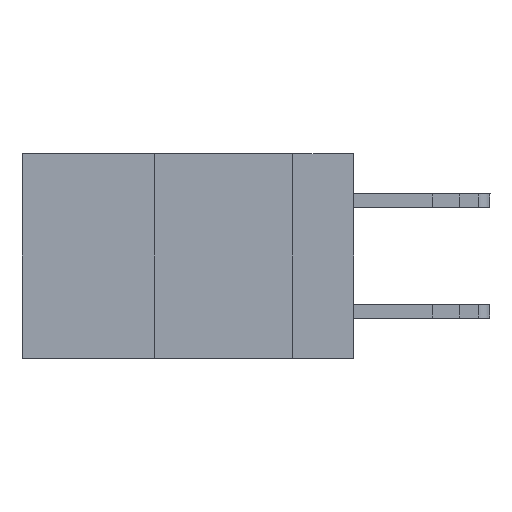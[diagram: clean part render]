
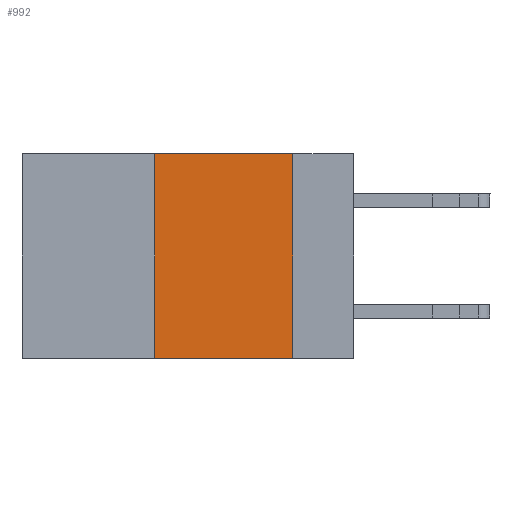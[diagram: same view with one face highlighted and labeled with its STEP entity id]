
A CAD part, left-side view. The second image highlights one B-rep face of the part: STEP entity #992.
In plain terms, the highlighted planar face has unit normal (-1, 0, 0).
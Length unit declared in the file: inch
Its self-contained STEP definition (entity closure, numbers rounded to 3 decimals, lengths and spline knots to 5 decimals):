
#744 = CARTESIAN_POINT ( 'NONE',  ( 0., 0.6, 0. ) ) ;
#855 = VERTEX_POINT ( 'NONE', #23430 ) ;
#992 = ADVANCED_FACE ( 'NONE', ( #20292 ), #3676, .F. ) ;
#1057 = LINE ( 'NONE', #10386, #12485 ) ;
#1118 = EDGE_CURVE ( 'NONE', #20044, #12864, #6195, .T. ) ;
#3676 = PLANE ( 'NONE',  #14341 ) ;
#4461 = LINE ( 'NONE', #11482, #5507 ) ;
#4913 = EDGE_CURVE ( 'NONE', #12864, #23146, #6655, .T. ) ;
#5507 = VECTOR ( 'NONE', #13796, 39.37008 ) ;
#6195 = LINE ( 'NONE', #744, #15088 ) ;
#6655 = LINE ( 'NONE', #12475, #9966 ) ;
#8420 = ORIENTED_EDGE ( 'NONE', *, *, #4913, .F. ) ;
#9239 = DIRECTION ( 'NONE',  ( 0., 0., -1. ) ) ;
#9966 = VECTOR ( 'NONE', #14059, 39.37008 ) ;
#10386 = CARTESIAN_POINT ( 'NONE',  ( 0., 0.36, 0. ) ) ;
#11059 = DIRECTION ( 'NONE',  ( 1., 0., 0. ) ) ;
#11482 = CARTESIAN_POINT ( 'NONE',  ( 0., 0.6, -0.37 ) ) ;
#11906 = EDGE_CURVE ( 'NONE', #855, #20044, #1057, .T. ) ;
#12475 = CARTESIAN_POINT ( 'NONE',  ( 0., 0.11, 0. ) ) ;
#12485 = VECTOR ( 'NONE', #14269, 39.37008 ) ;
#12864 = VERTEX_POINT ( 'NONE', #19680 ) ;
#13650 = ORIENTED_EDGE ( 'NONE', *, *, #1118, .F. ) ;
#13796 = DIRECTION ( 'NONE',  ( 0., -1., 0. ) ) ;
#14059 = DIRECTION ( 'NONE',  ( 0., 0., -1. ) ) ;
#14269 = DIRECTION ( 'NONE',  ( 0., 0., 1. ) ) ;
#14341 = AXIS2_PLACEMENT_3D ( 'NONE', #16759, #11059, #9239 ) ;
#15088 = VECTOR ( 'NONE', #15409, 39.37008 ) ;
#15409 = DIRECTION ( 'NONE',  ( 0., -1., 0. ) ) ;
#16759 = CARTESIAN_POINT ( 'NONE',  ( 0., 0.6, 0. ) ) ;
#16956 = ORIENTED_EDGE ( 'NONE', *, *, #23212, .T. ) ;
#18638 = CARTESIAN_POINT ( 'NONE',  ( 0., 0.36, 0. ) ) ;
#19680 = CARTESIAN_POINT ( 'NONE',  ( 0., 0.11, 0. ) ) ;
#20044 = VERTEX_POINT ( 'NONE', #18638 ) ;
#20240 = CARTESIAN_POINT ( 'NONE',  ( 0., 0.11, -0.37 ) ) ;
#20292 = FACE_OUTER_BOUND ( 'NONE', #20728, .T. ) ;
#20728 = EDGE_LOOP ( 'NONE', ( #8420, #13650, #23538, #16956 ) ) ;
#23146 = VERTEX_POINT ( 'NONE', #20240 ) ;
#23212 = EDGE_CURVE ( 'NONE', #855, #23146, #4461, .T. ) ;
#23430 = CARTESIAN_POINT ( 'NONE',  ( 0., 0.36, -0.37 ) ) ;
#23538 = ORIENTED_EDGE ( 'NONE', *, *, #11906, .F. ) ;
